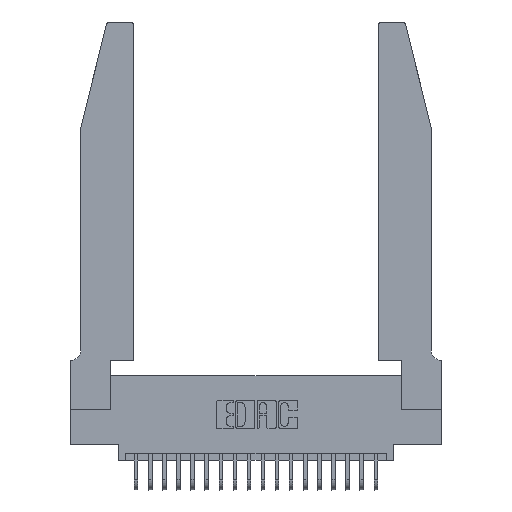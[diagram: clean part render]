
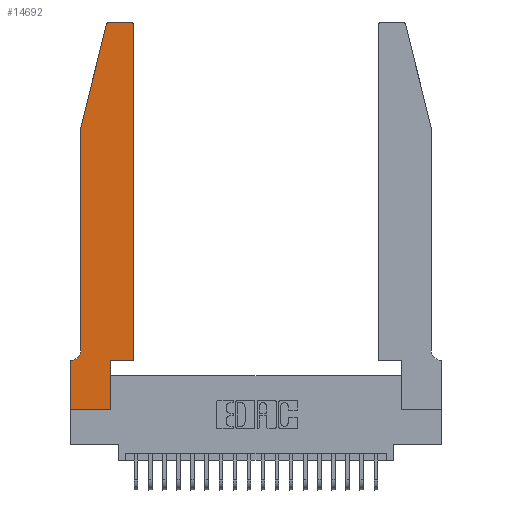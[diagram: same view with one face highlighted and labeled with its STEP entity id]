
A CAD part, top view. The second image highlights one B-rep face of the part: STEP entity #14692.
In plain terms, the highlighted planar face has unit normal (0, 0, 1).
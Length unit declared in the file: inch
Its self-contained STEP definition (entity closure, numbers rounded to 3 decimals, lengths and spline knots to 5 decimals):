
#70 = CARTESIAN_POINT ( 'NONE',  ( 0.0755, 2., 0.37 ) ) ;
#342 = CARTESIAN_POINT ( 'NONE',  ( 0.0755, 0.35, 0.37 ) ) ;
#352 = VERTEX_POINT ( 'NONE', #3524 ) ;
#405 = CARTESIAN_POINT ( 'NONE',  ( 0.0055, 0.35, 0.37 ) ) ;
#420 = CARTESIAN_POINT ( 'NONE',  ( 0.2865, 0.35, 0.37 ) ) ;
#1163 = ORIENTED_EDGE ( 'NONE', *, *, #11008, .T. ) ;
#1218 = ORIENTED_EDGE ( 'NONE', *, *, #20162, .T. ) ;
#1313 = EDGE_CURVE ( 'NONE', #12960, #2431, #3868, .T. ) ;
#1468 = CIRCLE ( 'NONE', #16898, 0.03 ) ;
#1783 = CARTESIAN_POINT ( 'NONE',  ( 0.2605, 2.75, 0.37 ) ) ;
#1805 = ORIENTED_EDGE ( 'NONE', *, *, #1313, .T. ) ;
#2207 = DIRECTION ( 'NONE',  ( 0., 1., 0. ) ) ;
#2357 = ORIENTED_EDGE ( 'NONE', *, *, #14053, .T. ) ;
#2431 = VERTEX_POINT ( 'NONE', #6517 ) ;
#2584 = DIRECTION ( 'NONE',  ( 0., 0., 1. ) ) ;
#2693 = VERTEX_POINT ( 'NONE', #7047 ) ;
#3354 = LINE ( 'NONE', #19272, #12029 ) ;
#3431 = DIRECTION ( 'NONE',  ( -1., 0., 0. ) ) ;
#3524 = CARTESIAN_POINT ( 'NONE',  ( 0.0755, 2., 0.37 ) ) ;
#3782 = CARTESIAN_POINT ( 'NONE',  ( 0., 0.35, 0.37 ) ) ;
#3868 = LINE ( 'NONE', #342, #12270 ) ;
#4080 = ORIENTED_EDGE ( 'NONE', *, *, #10773, .T. ) ;
#4201 = CIRCLE ( 'NONE', #6726, 0.03 ) ;
#4383 = VERTEX_POINT ( 'NONE', #21981 ) ;
#5136 = VECTOR ( 'NONE', #7570, 39.37008 ) ;
#5406 = EDGE_CURVE ( 'NONE', #13640, #4383, #4201, .T. ) ;
#6034 = VECTOR ( 'NONE', #14896, 39.37008 ) ;
#6088 = VERTEX_POINT ( 'NONE', #21654 ) ;
#6517 = CARTESIAN_POINT ( 'NONE',  ( 0., 0.35, 0.37 ) ) ;
#6641 = LINE ( 'NONE', #1783, #13584 ) ;
#6726 = AXIS2_PLACEMENT_3D ( 'NONE', #20400, #14872, #13108 ) ;
#6763 = LINE ( 'NONE', #420, #20109 ) ;
#7037 = VECTOR ( 'NONE', #13928, 39.37008 ) ;
#7047 = CARTESIAN_POINT ( 'NONE',  ( 0.4505, 0.35, 0.37 ) ) ;
#7155 = LINE ( 'NONE', #18646, #17010 ) ;
#7485 = CARTESIAN_POINT ( 'NONE',  ( 0., 0., 0.37 ) ) ;
#7570 = DIRECTION ( 'NONE',  ( 1., 0., 0. ) ) ;
#7751 = VECTOR ( 'NONE', #12809, 39.37008 ) ;
#7781 = DIRECTION ( 'NONE',  ( -1., 0., 0. ) ) ;
#8342 = ORIENTED_EDGE ( 'NONE', *, *, #14617, .T. ) ;
#8858 = EDGE_CURVE ( 'NONE', #2693, #23535, #3354, .T. ) ;
#9446 = DIRECTION ( 'NONE',  ( -0.239, -0.971, 0. ) ) ;
#9669 = DIRECTION ( 'NONE',  ( 0., 0., -1. ) ) ;
#9759 = VERTEX_POINT ( 'NONE', #12652 ) ;
#9794 = LINE ( 'NONE', #11307, #6034 ) ;
#10773 = EDGE_CURVE ( 'NONE', #20974, #23055, #6763, .T. ) ;
#10917 = DIRECTION ( 'NONE',  ( -1., 0., 0. ) ) ;
#11008 = EDGE_CURVE ( 'NONE', #2431, #6088, #13129, .T. ) ;
#11230 = CARTESIAN_POINT ( 'NONE',  ( 0.0055, 0.42, 0.37 ) ) ;
#11307 = CARTESIAN_POINT ( 'NONE',  ( 0.4505, 0.35, 0.37 ) ) ;
#11451 = VERTEX_POINT ( 'NONE', #11921 ) ;
#11481 = ORIENTED_EDGE ( 'NONE', *, *, #5406, .T. ) ;
#11921 = CARTESIAN_POINT ( 'NONE',  ( 0.4205, 2.75, 0.37 ) ) ;
#12029 = VECTOR ( 'NONE', #15379, 39.37008 ) ;
#12270 = VECTOR ( 'NONE', #3431, 39.37008 ) ;
#12331 = EDGE_LOOP ( 'NONE', ( #1218, #11481, #2357, #14158, #12710, #1805, #1163, #16125, #4080, #8342, #18728, #22648 ) ) ;
#12652 = CARTESIAN_POINT ( 'NONE',  ( 0.0755, 0.42, 0.37 ) ) ;
#12710 = ORIENTED_EDGE ( 'NONE', *, *, #12858, .T. ) ;
#12809 = DIRECTION ( 'NONE',  ( 0., -1., 0. ) ) ;
#12858 = EDGE_CURVE ( 'NONE', #9759, #12960, #23733, .T. ) ;
#12960 = VERTEX_POINT ( 'NONE', #405 ) ;
#13108 = DIRECTION ( 'NONE',  ( 1., 0., 0. ) ) ;
#13129 = LINE ( 'NONE', #23403, #7037 ) ;
#13264 = LINE ( 'NONE', #70, #7751 ) ;
#13584 = VECTOR ( 'NONE', #10917, 39.37008 ) ;
#13640 = VERTEX_POINT ( 'NONE', #15517 ) ;
#13928 = DIRECTION ( 'NONE',  ( 0., -1., 0. ) ) ;
#14053 = EDGE_CURVE ( 'NONE', #4383, #352, #7155, .T. ) ;
#14158 = ORIENTED_EDGE ( 'NONE', *, *, #21107, .T. ) ;
#14617 = EDGE_CURVE ( 'NONE', #23055, #2693, #9794, .T. ) ;
#14692 = ADVANCED_FACE ( 'NONE', ( #19025 ), #14813, .T. ) ;
#14813 = PLANE ( 'NONE',  #20971 ) ;
#14872 = DIRECTION ( 'NONE',  ( 0., 0., 1. ) ) ;
#14896 = DIRECTION ( 'NONE',  ( 1., 0., 0. ) ) ;
#14946 = LINE ( 'NONE', #7485, #5136 ) ;
#15379 = DIRECTION ( 'NONE',  ( 0., 1., 0. ) ) ;
#15470 = EDGE_CURVE ( 'NONE', #6088, #20974, #14946, .T. ) ;
#15517 = CARTESIAN_POINT ( 'NONE',  ( 0.284, 2.75, 0.37 ) ) ;
#16125 = ORIENTED_EDGE ( 'NONE', *, *, #15470, .T. ) ;
#16331 = CARTESIAN_POINT ( 'NONE',  ( 0.4505, 2.72, 0.37 ) ) ;
#16694 = DIRECTION ( 'NONE',  ( 1., 0., 0. ) ) ;
#16898 = AXIS2_PLACEMENT_3D ( 'NONE', #22911, #2584, #19189 ) ;
#17010 = VECTOR ( 'NONE', #9446, 39.37008 ) ;
#17995 = AXIS2_PLACEMENT_3D ( 'NONE', #11230, #9669, #7781 ) ;
#18372 = CARTESIAN_POINT ( 'NONE',  ( 0.2865, 0.35, 0.37 ) ) ;
#18378 = CARTESIAN_POINT ( 'NONE',  ( 0.2865, 0., 0.37 ) ) ;
#18646 = CARTESIAN_POINT ( 'NONE',  ( 0.0755, 2., 0.37 ) ) ;
#18728 = ORIENTED_EDGE ( 'NONE', *, *, #8858, .T. ) ;
#19025 = FACE_OUTER_BOUND ( 'NONE', #12331, .T. ) ;
#19189 = DIRECTION ( 'NONE',  ( 1., 0., 0. ) ) ;
#19272 = CARTESIAN_POINT ( 'NONE',  ( 0.4505, 0.35, 0.37 ) ) ;
#20109 = VECTOR ( 'NONE', #2207, 39.37008 ) ;
#20162 = EDGE_CURVE ( 'NONE', #11451, #13640, #6641, .T. ) ;
#20400 = CARTESIAN_POINT ( 'NONE',  ( 0.284, 2.72, 0.37 ) ) ;
#20439 = EDGE_CURVE ( 'NONE', #23535, #11451, #1468, .T. ) ;
#20580 = DIRECTION ( 'NONE',  ( 0., 0., 1. ) ) ;
#20971 = AXIS2_PLACEMENT_3D ( 'NONE', #3782, #20580, #16694 ) ;
#20974 = VERTEX_POINT ( 'NONE', #18378 ) ;
#21107 = EDGE_CURVE ( 'NONE', #352, #9759, #13264, .T. ) ;
#21654 = CARTESIAN_POINT ( 'NONE',  ( 0., 0., 0.37 ) ) ;
#21981 = CARTESIAN_POINT ( 'NONE',  ( 0.25487, 2.72718, 0.37 ) ) ;
#22648 = ORIENTED_EDGE ( 'NONE', *, *, #20439, .T. ) ;
#22911 = CARTESIAN_POINT ( 'NONE',  ( 0.4205, 2.72, 0.37 ) ) ;
#23055 = VERTEX_POINT ( 'NONE', #18372 ) ;
#23403 = CARTESIAN_POINT ( 'NONE',  ( 0., 0., 0.37 ) ) ;
#23535 = VERTEX_POINT ( 'NONE', #16331 ) ;
#23733 = CIRCLE ( 'NONE', #17995, 0.07 ) ;
